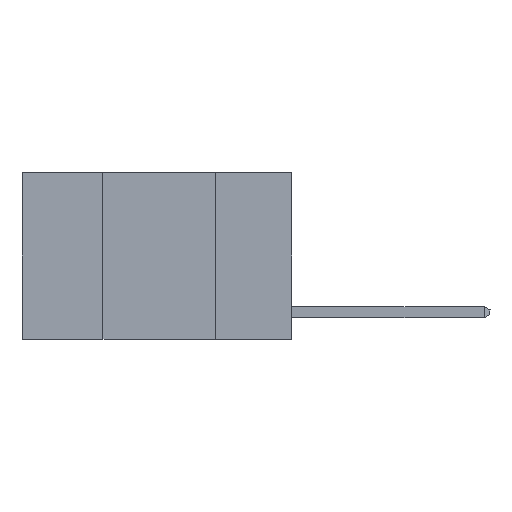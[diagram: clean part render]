
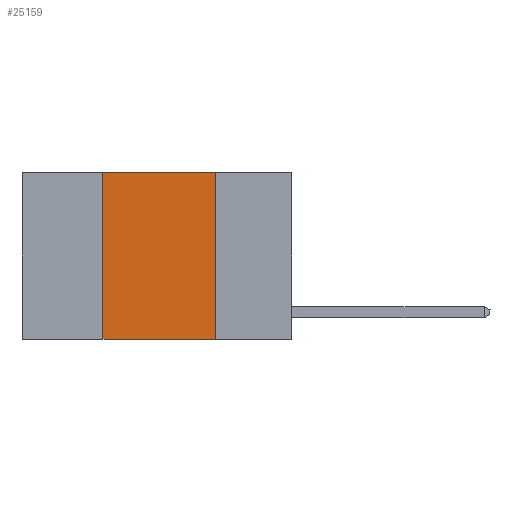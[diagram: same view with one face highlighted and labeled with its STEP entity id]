
A CAD part, left-side view. The second image highlights one B-rep face of the part: STEP entity #25159.
In plain terms, the highlighted planar face has unit normal (-1, 0, 0).
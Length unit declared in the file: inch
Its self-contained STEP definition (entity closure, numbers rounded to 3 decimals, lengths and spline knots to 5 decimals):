
#1395 = LINE ( 'NONE', #13547, #23934 ) ;
#1439 = CARTESIAN_POINT ( 'NONE',  ( 0., 0.6, 0. ) ) ;
#1524 = DIRECTION ( 'NONE',  ( 1., 0., 0. ) ) ;
#2213 = CARTESIAN_POINT ( 'NONE',  ( 0., 0.42, 0. ) ) ;
#2358 = DIRECTION ( 'NONE',  ( 0., -1., 0. ) ) ;
#4885 = DIRECTION ( 'NONE',  ( 0., -1., 0. ) ) ;
#5519 = EDGE_CURVE ( 'NONE', #27765, #24284, #17208, .T. ) ;
#6076 = CARTESIAN_POINT ( 'NONE',  ( 0., 0.17, -0.37 ) ) ;
#6461 = EDGE_CURVE ( 'NONE', #25571, #24284, #1395, .T. ) ;
#8680 = ORIENTED_EDGE ( 'NONE', *, *, #15070, .F. ) ;
#9333 = ORIENTED_EDGE ( 'NONE', *, *, #6461, .T. ) ;
#10449 = AXIS2_PLACEMENT_3D ( 'NONE', #1439, #1524, #16798 ) ;
#12335 = FACE_OUTER_BOUND ( 'NONE', #13054, .T. ) ;
#13054 = EDGE_LOOP ( 'NONE', ( #26279, #8680, #16443, #9333 ) ) ;
#13255 = CARTESIAN_POINT ( 'NONE',  ( 0., 0.6, 0. ) ) ;
#13547 = CARTESIAN_POINT ( 'NONE',  ( 0., 0.6, -0.37 ) ) ;
#14747 = DIRECTION ( 'NONE',  ( 0., 0., -1. ) ) ;
#15070 = EDGE_CURVE ( 'NONE', #27088, #27765, #27549, .T. ) ;
#16044 = VECTOR ( 'NONE', #2358, 39.37008 ) ;
#16443 = ORIENTED_EDGE ( 'NONE', *, *, #22453, .F. ) ;
#16524 = VECTOR ( 'NONE', #14747, 39.37008 ) ;
#16798 = DIRECTION ( 'NONE',  ( 0., 0., -1. ) ) ;
#16887 = CARTESIAN_POINT ( 'NONE',  ( 0., 0.17, 0. ) ) ;
#17208 = LINE ( 'NONE', #16887, #16524 ) ;
#17474 = DIRECTION ( 'NONE',  ( 0., 0., 1. ) ) ;
#20293 = CARTESIAN_POINT ( 'NONE',  ( 0., 0.42, -0.37 ) ) ;
#21470 = CARTESIAN_POINT ( 'NONE',  ( 0., 0.42, 0. ) ) ;
#22453 = EDGE_CURVE ( 'NONE', #25571, #27088, #27760, .T. ) ;
#22712 = VECTOR ( 'NONE', #17474, 39.37008 ) ;
#23934 = VECTOR ( 'NONE', #4885, 39.37008 ) ;
#24284 = VERTEX_POINT ( 'NONE', #6076 ) ;
#25159 = ADVANCED_FACE ( 'NONE', ( #12335 ), #25451, .F. ) ;
#25451 = PLANE ( 'NONE',  #10449 ) ;
#25571 = VERTEX_POINT ( 'NONE', #20293 ) ;
#26279 = ORIENTED_EDGE ( 'NONE', *, *, #5519, .F. ) ;
#27088 = VERTEX_POINT ( 'NONE', #21470 ) ;
#27549 = LINE ( 'NONE', #13255, #16044 ) ;
#27760 = LINE ( 'NONE', #2213, #22712 ) ;
#27765 = VERTEX_POINT ( 'NONE', #28117 ) ;
#28117 = CARTESIAN_POINT ( 'NONE',  ( 0., 0.17, 0. ) ) ;
